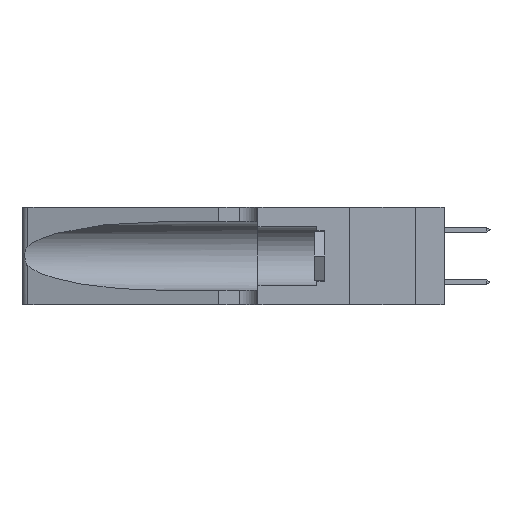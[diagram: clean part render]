
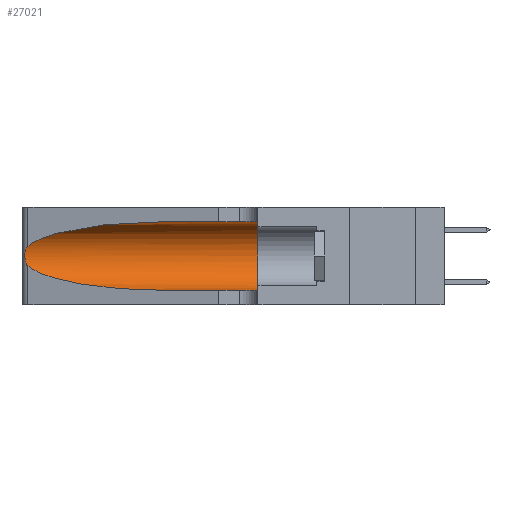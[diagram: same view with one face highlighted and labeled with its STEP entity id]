
A CAD part, left-side view. The second image highlights one B-rep face of the part: STEP entity #27021.
In plain terms, the highlighted cylindrical face has radius 3.308 mm (diameter 6.617 mm), a partial arc.
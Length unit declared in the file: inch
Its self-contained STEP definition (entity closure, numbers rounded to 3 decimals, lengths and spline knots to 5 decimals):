
#41 = CARTESIAN_POINT ( 'NONE',  ( 0.26075, 1.23896, 0.19203 ) ) ;
#179 = DIRECTION ( 'NONE',  ( 0., -1., 0. ) ) ;
#1488 = CARTESIAN_POINT ( 'NONE',  ( 0.1305, 1.61858, 0.31525 ) ) ;
#1823 = CARTESIAN_POINT ( 'NONE',  ( 0.25487, 1.22718, 0.14631 ) ) ;
#1951 = ORIENTED_EDGE ( 'NONE', *, *, #30776, .T. ) ;
#1992 = VECTOR ( 'NONE', #179, 39.37008 ) ;
#2044 = EDGE_CURVE ( 'NONE', #29743, #18941, #33166, .T. ) ;
#2218 = VERTEX_POINT ( 'NONE', #28615 ) ;
#2223 = AXIS2_PLACEMENT_3D ( 'NONE', #6457, #15185, #6730 ) ;
#2764 = EDGE_LOOP ( 'NONE', ( #31528, #17422, #1951, #3260, #37352, #11028 ) ) ;
#2843 = VECTOR ( 'NONE', #25136, 39.37008 ) ;
#3260 = ORIENTED_EDGE ( 'NONE', *, *, #2044, .T. ) ;
#5836 = CARTESIAN_POINT ( 'NONE',  ( 0.1305, 0.72297, 0.05475 ) ) ;
#6457 = CARTESIAN_POINT ( 'NONE',  ( 0.1305, 1.61858, 0.185 ) ) ;
#6730 = DIRECTION ( 'NONE',  ( 0., 0., -1. ) ) ;
#6978 = CYLINDRICAL_SURFACE ( 'NONE', #2223, 0.13025 ) ;
#7500 = VERTEX_POINT ( 'NONE', #1823 ) ;
#8859 = CARTESIAN_POINT ( 'NONE',  ( 0.25555, 1.22993, 0.14849 ) ) ;
#10865 = CARTESIAN_POINT ( 'NONE',  ( 0.2373, 1.15595, 0.28018 ) ) ;
#10989 = CARTESIAN_POINT ( 'NONE',  ( 0.18966, 0.96281, 0.31525 ) ) ;
#11028 = ORIENTED_EDGE ( 'NONE', *, *, #27091, .F. ) ;
#11271 =( BOUNDED_CURVE ( )  B_SPLINE_CURVE ( 3, ( #22363, #28252, #34137, #33880 ),
 .UNSPECIFIED., .F., .F. ) 
 B_SPLINE_CURVE_WITH_KNOTS ( ( 4, 4 ),
 ( 3.44316, 4.71239 ),
 .UNSPECIFIED. ) 
 CURVE ( )  GEOMETRIC_REPRESENTATION_ITEM ( )  RATIONAL_B_SPLINE_CURVE ( ( 1., 0.87, 0.87, 1. ) ) 
 REPRESENTATION_ITEM ( '' )  );
#11448 = CARTESIAN_POINT ( 'NONE',  ( 0.25854, 1.2359, 0.20912 ) ) ;
#11636 = CARTESIAN_POINT ( 'NONE',  ( 0.1305, 0.72297, 0.31525 ) ) ;
#13256 = CARTESIAN_POINT ( 'NONE',  ( 0.1305, 0.35, 0.31525 ) ) ;
#14551 = CARTESIAN_POINT ( 'NONE',  ( 0.26075, 1.23896, 0.178 ) ) ;
#14780 = CARTESIAN_POINT ( 'NONE',  ( 0.25856, 1.23593, 0.16098 ) ) ;
#14900 = CARTESIAN_POINT ( 'NONE',  ( 0.25639, 1.23186, 0.15144 ) ) ;
#15185 = DIRECTION ( 'NONE',  ( 0., -1., 0. ) ) ;
#17422 = ORIENTED_EDGE ( 'NONE', *, *, #33568, .T. ) ;
#18941 = VERTEX_POINT ( 'NONE', #21120 ) ;
#19722 = CARTESIAN_POINT ( 'NONE',  ( 0.25787, 1.23484, 0.2124 ) ) ;
#19766 = CARTESIAN_POINT ( 'NONE',  ( 0.1305, 0.72297, 0.31525 ) ) ;
#21120 = CARTESIAN_POINT ( 'NONE',  ( 0.1305, 0.35, 0.05475 ) ) ;
#21131 = DIRECTION ( 'NONE',  ( 0., 1., 0. ) ) ;
#22363 = CARTESIAN_POINT ( 'NONE',  ( 0.25487, 1.22718, 0.14631 ) ) ;
#22533 = CARTESIAN_POINT ( 'NONE',  ( 0.25487, 1.22718, 0.22369 ) ) ;
#22834 = B_SPLINE_CURVE_WITH_KNOTS ( 'NONE', 3,
 ( #22533, #31342, #37240, #19722, #11448, #29550, #41, #14551, #23420, #14780, #26490, #14900, #8859, #35286 ),
 .UNSPECIFIED., .F., .F.,
 ( 4, 2, 2, 2, 2, 2, 4 ),
 ( 0., 0.00027, 0.00053, 0.00107, 0.0016, 0.00187, 0.00214 ),
 .UNSPECIFIED. ) ;
#22841 = EDGE_CURVE ( 'NONE', #32342, #2218, #32872, .T. ) ;
#23420 = CARTESIAN_POINT ( 'NONE',  ( 0.26017, 1.23833, 0.17102 ) ) ;
#25136 = DIRECTION ( 'NONE',  ( 0., -1., 0. ) ) ;
#25368 = LINE ( 'NONE', #1488, #2843 ) ;
#26490 = CARTESIAN_POINT ( 'NONE',  ( 0.25789, 1.23486, 0.15765 ) ) ;
#27021 = ADVANCED_FACE ( 'NONE', ( #34968 ), #6978, .F. ) ;
#27091 = EDGE_CURVE ( 'NONE', #32342, #34547, #25368, .T. ) ;
#27256 = AXIS2_PLACEMENT_3D ( 'NONE', #35710, #21131, #35837 ) ;
#28252 = CARTESIAN_POINT ( 'NONE',  ( 0.2373, 1.15595, 0.08982 ) ) ;
#28615 = CARTESIAN_POINT ( 'NONE',  ( 0.25487, 1.22718, 0.22369 ) ) ;
#29550 = CARTESIAN_POINT ( 'NONE',  ( 0.26018, 1.23835, 0.19895 ) ) ;
#29743 = VERTEX_POINT ( 'NONE', #5836 ) ;
#29800 = CARTESIAN_POINT ( 'NONE',  ( 0.1305, 1.61858, 0.05475 ) ) ;
#30776 = EDGE_CURVE ( 'NONE', #7500, #29743, #11271, .T. ) ;
#31342 = CARTESIAN_POINT ( 'NONE',  ( 0.25555, 1.22994, 0.2215 ) ) ;
#31528 = ORIENTED_EDGE ( 'NONE', *, *, #22841, .T. ) ;
#32342 = VERTEX_POINT ( 'NONE', #11636 ) ;
#32872 =( BOUNDED_CURVE ( )  B_SPLINE_CURVE ( 3, ( #19766, #10989, #10865, #37674 ),
 .UNSPECIFIED., .F., .F. ) 
 B_SPLINE_CURVE_WITH_KNOTS ( ( 4, 4 ),
 ( 1.5708, 2.84003 ),
 .UNSPECIFIED. ) 
 CURVE ( )  GEOMETRIC_REPRESENTATION_ITEM ( )  RATIONAL_B_SPLINE_CURVE ( ( 1., 0.87, 0.87, 1. ) ) 
 REPRESENTATION_ITEM ( '' )  );
#33166 = LINE ( 'NONE', #29800, #1992 ) ;
#33568 = EDGE_CURVE ( 'NONE', #2218, #7500, #22834, .T. ) ;
#33880 = CARTESIAN_POINT ( 'NONE',  ( 0.1305, 0.72297, 0.05475 ) ) ;
#34137 = CARTESIAN_POINT ( 'NONE',  ( 0.18966, 0.96281, 0.05475 ) ) ;
#34547 = VERTEX_POINT ( 'NONE', #13256 ) ;
#34968 = FACE_OUTER_BOUND ( 'NONE', #2764, .T. ) ;
#35286 = CARTESIAN_POINT ( 'NONE',  ( 0.25487, 1.22718, 0.14631 ) ) ;
#35710 = CARTESIAN_POINT ( 'NONE',  ( 0.1305, 0.35, 0.185 ) ) ;
#35837 = DIRECTION ( 'NONE',  ( 0., 0., 1. ) ) ;
#35847 = CIRCLE ( 'NONE', #27256, 0.13025 ) ;
#37240 = CARTESIAN_POINT ( 'NONE',  ( 0.25639, 1.23184, 0.21858 ) ) ;
#37352 = ORIENTED_EDGE ( 'NONE', *, *, #37736, .F. ) ;
#37674 = CARTESIAN_POINT ( 'NONE',  ( 0.25487, 1.22718, 0.22369 ) ) ;
#37736 = EDGE_CURVE ( 'NONE', #34547, #18941, #35847, .T. ) ;
